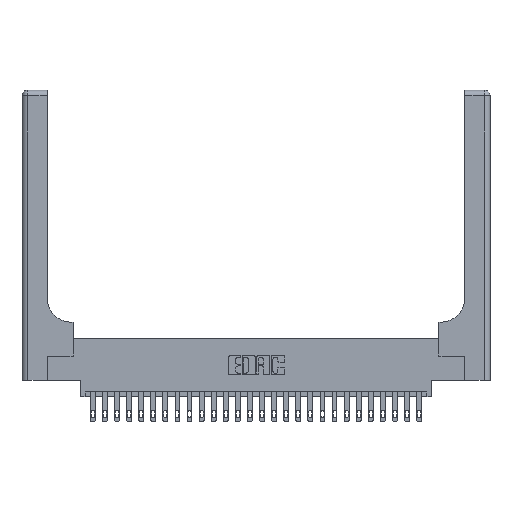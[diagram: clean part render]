
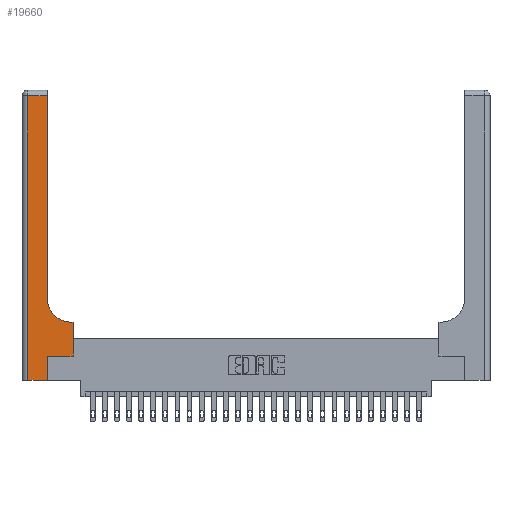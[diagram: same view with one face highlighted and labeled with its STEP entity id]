
A CAD part, top view. The second image highlights one B-rep face of the part: STEP entity #19660.
In plain terms, the highlighted planar face has unit normal (0, 0, 1).
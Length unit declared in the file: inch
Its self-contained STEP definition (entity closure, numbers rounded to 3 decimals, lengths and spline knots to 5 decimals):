
#449 = CARTESIAN_POINT ( 'NONE',  ( 0.528, 0.6, 0.37 ) ) ;
#608 = VERTEX_POINT ( 'NONE', #6808 ) ;
#853 = DIRECTION ( 'NONE',  ( 0., 1., 0. ) ) ;
#1685 = LINE ( 'NONE', #9685, #25404 ) ;
#1724 = CARTESIAN_POINT ( 'NONE',  ( 0.06, 0., 0.37 ) ) ;
#1825 = CARTESIAN_POINT ( 'NONE',  ( 0.26, 0.6, 0.37 ) ) ;
#1883 = CARTESIAN_POINT ( 'NONE',  ( 0.51, 0.85, 0.37 ) ) ;
#1923 = VECTOR ( 'NONE', #23638, 39.37008 ) ;
#1942 = CARTESIAN_POINT ( 'NONE',  ( 0.06, 2.94, 0.37 ) ) ;
#2263 = ORIENTED_EDGE ( 'NONE', *, *, #22558, .T. ) ;
#2954 = CIRCLE ( 'NONE', #5012, 0.25 ) ;
#3518 = DIRECTION ( 'NONE',  ( 0., 0., -1. ) ) ;
#3601 = DIRECTION ( 'NONE',  ( 0., 0., -1. ) ) ;
#3829 = LINE ( 'NONE', #10366, #6464 ) ;
#3836 = VERTEX_POINT ( 'NONE', #13957 ) ;
#4608 = ORIENTED_EDGE ( 'NONE', *, *, #14346, .T. ) ;
#4933 = VECTOR ( 'NONE', #16951, 39.37008 ) ;
#4934 = ORIENTED_EDGE ( 'NONE', *, *, #24740, .T. ) ;
#5012 = AXIS2_PLACEMENT_3D ( 'NONE', #1883, #3601, #5709 ) ;
#5059 = EDGE_CURVE ( 'NONE', #608, #13911, #2954, .T. ) ;
#5329 = LINE ( 'NONE', #15543, #1923 ) ;
#5547 = ORIENTED_EDGE ( 'NONE', *, *, #18754, .T. ) ;
#5584 = VECTOR ( 'NONE', #853, 39.37008 ) ;
#5709 = DIRECTION ( 'NONE',  ( 1., 0., 0. ) ) ;
#5766 = CARTESIAN_POINT ( 'NONE',  ( 0., 0., 0.37 ) ) ;
#6464 = VECTOR ( 'NONE', #24372, 39.37008 ) ;
#6523 = EDGE_LOOP ( 'NONE', ( #6920, #4934, #5547, #19893, #4608, #2263, #21215, #16517, #25078 ) ) ;
#6808 = CARTESIAN_POINT ( 'NONE',  ( 0.51, 0.6, 0.37 ) ) ;
#6920 = ORIENTED_EDGE ( 'NONE', *, *, #15406, .T. ) ;
#7213 = DIRECTION ( 'NONE',  ( 1., 0., 0. ) ) ;
#8842 = LINE ( 'NONE', #22842, #5584 ) ;
#9131 = VERTEX_POINT ( 'NONE', #17115 ) ;
#9604 = EDGE_CURVE ( 'NONE', #15566, #15057, #20720, .T. ) ;
#9685 = CARTESIAN_POINT ( 'NONE',  ( 0.265, 0.25, 0.37 ) ) ;
#9746 = VERTEX_POINT ( 'NONE', #1724 ) ;
#10366 = CARTESIAN_POINT ( 'NONE',  ( 0.26, 3., 0.37 ) ) ;
#11635 = FACE_OUTER_BOUND ( 'NONE', #6523, .T. ) ;
#12669 = CARTESIAN_POINT ( 'NONE',  ( 0.26, 0.85, 0.37 ) ) ;
#13621 = CARTESIAN_POINT ( 'NONE',  ( 0., 3., 0.37 ) ) ;
#13684 = VERTEX_POINT ( 'NONE', #1942 ) ;
#13687 = LINE ( 'NONE', #21903, #20454 ) ;
#13806 = CARTESIAN_POINT ( 'NONE',  ( 0.265, 0.25, 0.37 ) ) ;
#13911 = VERTEX_POINT ( 'NONE', #12669 ) ;
#13957 = CARTESIAN_POINT ( 'NONE',  ( 0.265, 0., 0.37 ) ) ;
#14346 = EDGE_CURVE ( 'NONE', #3836, #15405, #8842, .T. ) ;
#15057 = VERTEX_POINT ( 'NONE', #449 ) ;
#15405 = VERTEX_POINT ( 'NONE', #13806 ) ;
#15406 = EDGE_CURVE ( 'NONE', #13911, #9131, #3829, .T. ) ;
#15543 = CARTESIAN_POINT ( 'NONE',  ( 0.06, 3., 0.37 ) ) ;
#15566 = VERTEX_POINT ( 'NONE', #25146 ) ;
#15739 = EDGE_CURVE ( 'NONE', #15057, #608, #23694, .T. ) ;
#15835 = DIRECTION ( 'NONE',  ( -1., 0., 0. ) ) ;
#16517 = ORIENTED_EDGE ( 'NONE', *, *, #15739, .T. ) ;
#16951 = DIRECTION ( 'NONE',  ( 0., 1., 0. ) ) ;
#17115 = CARTESIAN_POINT ( 'NONE',  ( 0.26, 2.94, 0.37 ) ) ;
#17419 = PLANE ( 'NONE',  #19936 ) ;
#17695 = DIRECTION ( 'NONE',  ( 1., 0., 0. ) ) ;
#18754 = EDGE_CURVE ( 'NONE', #13684, #9746, #5329, .T. ) ;
#19660 = ADVANCED_FACE ( 'NONE', ( #11635 ), #17419, .F. ) ;
#19893 = ORIENTED_EDGE ( 'NONE', *, *, #25472, .T. ) ;
#19936 = AXIS2_PLACEMENT_3D ( 'NONE', #13621, #3518, #15835 ) ;
#20454 = VECTOR ( 'NONE', #21388, 39.37008 ) ;
#20720 = LINE ( 'NONE', #24920, #4933 ) ;
#20830 = VECTOR ( 'NONE', #25537, 39.37008 ) ;
#21194 = LINE ( 'NONE', #5766, #22568 ) ;
#21215 = ORIENTED_EDGE ( 'NONE', *, *, #9604, .T. ) ;
#21388 = DIRECTION ( 'NONE',  ( -1., 0., 0. ) ) ;
#21903 = CARTESIAN_POINT ( 'NONE',  ( 0., 2.94, 0.37 ) ) ;
#22558 = EDGE_CURVE ( 'NONE', #15405, #15566, #1685, .T. ) ;
#22568 = VECTOR ( 'NONE', #7213, 39.37008 ) ;
#22842 = CARTESIAN_POINT ( 'NONE',  ( 0.265, 0., 0.37 ) ) ;
#23638 = DIRECTION ( 'NONE',  ( 0., -1., 0. ) ) ;
#23694 = LINE ( 'NONE', #1825, #20830 ) ;
#24372 = DIRECTION ( 'NONE',  ( 0., 1., 0. ) ) ;
#24740 = EDGE_CURVE ( 'NONE', #9131, #13684, #13687, .T. ) ;
#24920 = CARTESIAN_POINT ( 'NONE',  ( 0.528, 0.25, 0.37 ) ) ;
#25078 = ORIENTED_EDGE ( 'NONE', *, *, #5059, .T. ) ;
#25146 = CARTESIAN_POINT ( 'NONE',  ( 0.528, 0.25, 0.37 ) ) ;
#25404 = VECTOR ( 'NONE', #17695, 39.37008 ) ;
#25472 = EDGE_CURVE ( 'NONE', #9746, #3836, #21194, .T. ) ;
#25537 = DIRECTION ( 'NONE',  ( -1., 0., 0. ) ) ;
